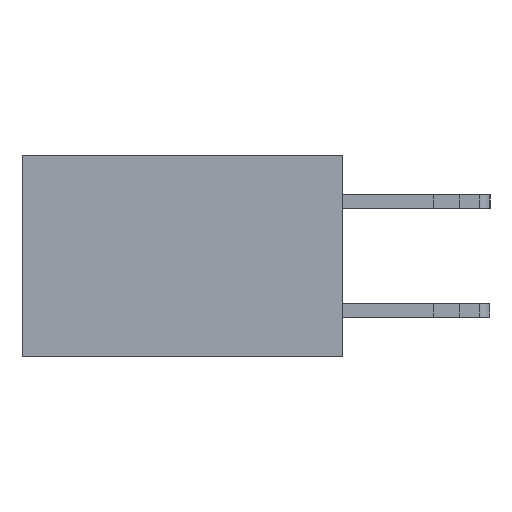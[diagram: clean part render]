
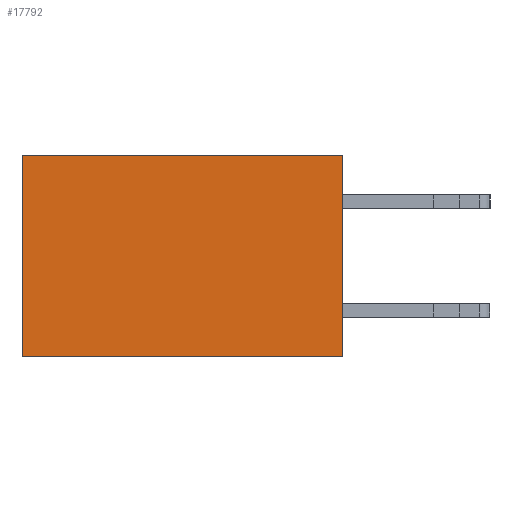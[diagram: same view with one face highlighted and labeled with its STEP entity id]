
A CAD part, left-side view. The second image highlights one B-rep face of the part: STEP entity #17792.
In plain terms, the highlighted planar face has unit normal (-1, 0, 0).
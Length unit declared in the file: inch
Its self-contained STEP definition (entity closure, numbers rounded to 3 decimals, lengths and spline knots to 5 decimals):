
#730 = VERTEX_POINT ( 'NONE', #10275 ) ;
#2672 = DIRECTION ( 'NONE',  ( 0., 0., -1. ) ) ;
#2903 = CARTESIAN_POINT ( 'NONE',  ( 0.277, 0., -0.37 ) ) ;
#3478 = VECTOR ( 'NONE', #5760, 39.37008 ) ;
#4687 = EDGE_CURVE ( 'NONE', #19358, #9185, #12532, .T. ) ;
#5646 = EDGE_CURVE ( 'NONE', #14145, #730, #7798, .T. ) ;
#5760 = DIRECTION ( 'NONE',  ( 0., 1., 0. ) ) ;
#6746 = ORIENTED_EDGE ( 'NONE', *, *, #4687, .F. ) ;
#7294 = ORIENTED_EDGE ( 'NONE', *, *, #21029, .F. ) ;
#7688 = AXIS2_PLACEMENT_3D ( 'NONE', #17863, #12893, #2672 ) ;
#7798 = LINE ( 'NONE', #19219, #8322 ) ;
#7821 = PLANE ( 'NONE',  #7688 ) ;
#8322 = VECTOR ( 'NONE', #19247, 39.37008 ) ;
#8425 = LINE ( 'NONE', #10205, #16814 ) ;
#8521 = DIRECTION ( 'NONE',  ( 0., 0., -1. ) ) ;
#9185 = VERTEX_POINT ( 'NONE', #21577 ) ;
#10205 = CARTESIAN_POINT ( 'NONE',  ( 0.277, 0., -0.37 ) ) ;
#10275 = CARTESIAN_POINT ( 'NONE',  ( 0.277, 0.59, 0. ) ) ;
#11680 = VECTOR ( 'NONE', #14860, 39.37008 ) ;
#11758 = CARTESIAN_POINT ( 'NONE',  ( 0.277, 0., 0. ) ) ;
#12532 = LINE ( 'NONE', #2903, #3478 ) ;
#12876 = EDGE_LOOP ( 'NONE', ( #19587, #6746, #7294, #20395 ) ) ;
#12893 = DIRECTION ( 'NONE',  ( 1., 0., 0. ) ) ;
#13201 = CARTESIAN_POINT ( 'NONE',  ( 0.277, 0.59, -0.37 ) ) ;
#13251 = CARTESIAN_POINT ( 'NONE',  ( 0.277, 0., -0.37 ) ) ;
#14145 = VERTEX_POINT ( 'NONE', #11758 ) ;
#14649 = EDGE_CURVE ( 'NONE', #730, #9185, #16632, .T. ) ;
#14860 = DIRECTION ( 'NONE',  ( 0., 0., -1. ) ) ;
#15721 = FACE_OUTER_BOUND ( 'NONE', #12876, .T. ) ;
#16632 = LINE ( 'NONE', #13201, #11680 ) ;
#16814 = VECTOR ( 'NONE', #8521, 39.37008 ) ;
#17792 = ADVANCED_FACE ( 'NONE', ( #15721 ), #7821, .F. ) ;
#17863 = CARTESIAN_POINT ( 'NONE',  ( 0.277, 0., -0.37 ) ) ;
#19219 = CARTESIAN_POINT ( 'NONE',  ( 0.277, 0., 0. ) ) ;
#19247 = DIRECTION ( 'NONE',  ( 0., 1., 0. ) ) ;
#19358 = VERTEX_POINT ( 'NONE', #13251 ) ;
#19587 = ORIENTED_EDGE ( 'NONE', *, *, #14649, .T. ) ;
#20395 = ORIENTED_EDGE ( 'NONE', *, *, #5646, .T. ) ;
#21029 = EDGE_CURVE ( 'NONE', #14145, #19358, #8425, .T. ) ;
#21577 = CARTESIAN_POINT ( 'NONE',  ( 0.277, 0.59, -0.37 ) ) ;
